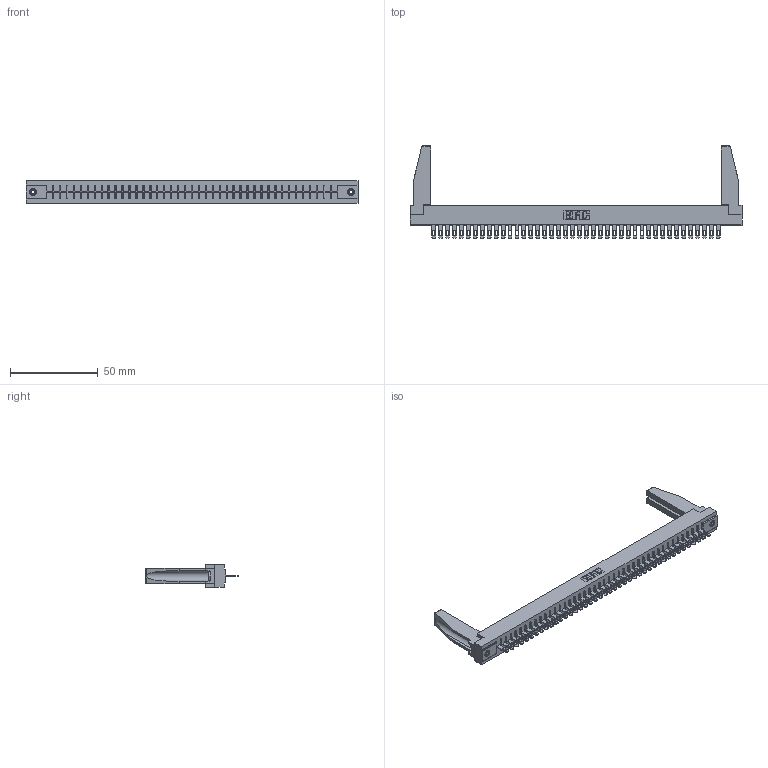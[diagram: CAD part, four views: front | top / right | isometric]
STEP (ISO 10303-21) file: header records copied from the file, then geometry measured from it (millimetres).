
FILE_DESCRIPTION (( 'STEP AP203' ), '1' );
FILE_NAME ('316-042-400-178.STEP', '2020-09-23T07:29:27', ( '' ), ( '' ), 'SwSTEP 2.0', 'SolidWorks 2020', '' );
FILE_SCHEMA (( 'CONFIG_CONTROL_DESIGN' ));
Length unit declared in the file: inch
Products named in the file (5): 316-042-400-178; 306 Part_.156 Dia; 306-290-001_100; 345-250-001_345-250-001-102; 307-220-078
Assembly tree (47 placements, depth 2):
  316-042-400-178
    306 Part_.156 Dia
    306-290-001_100  x42
    345-250-001_345-250-001-102  x2
    307-220-078  x2
Bounding box: 189.43 x 52.91 x 12.7 mm (x, y, z)
Volume: 25085.9 mm3; surface area: 26207.1 mm2
Topology: 47 solids, 47 shells, 3438 faces, 9676 edges, 6216 vertices
Faces by surface type: plane 2252, cylinder 1002, sphere 168, cone 12, torus 4
Entity records: 41770 total; most frequent: CARTESIAN_POINT 7015, ORIENTED_EDGE 6914, DIRECTION 6869, EDGE_CURVE 3457, VECTOR 2705, LINE 2705, VERTEX_POINT 2186, AXIS2_PLACEMENT_3D 2082
